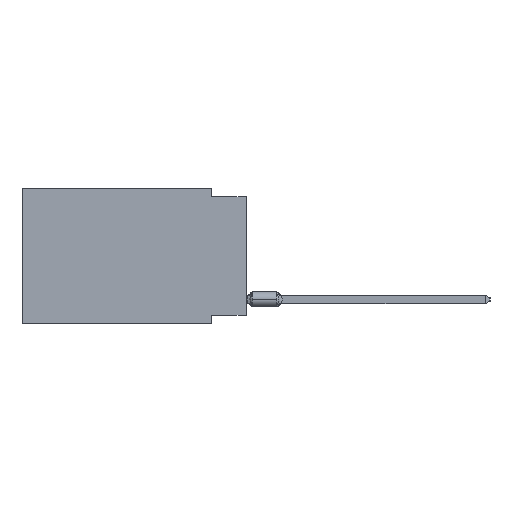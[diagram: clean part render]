
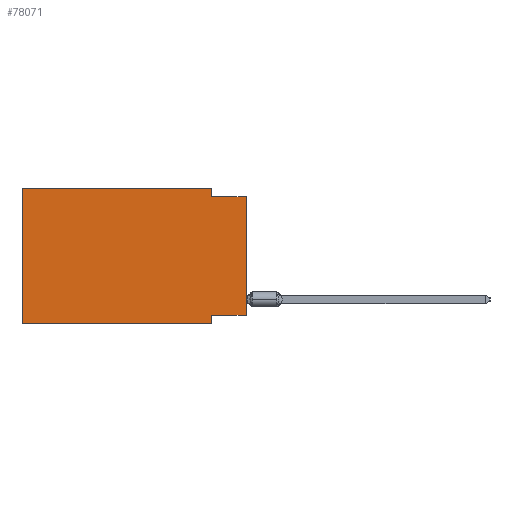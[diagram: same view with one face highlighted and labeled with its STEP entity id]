
A CAD part, left-side view. The second image highlights one B-rep face of the part: STEP entity #78071.
In plain terms, the highlighted planar face has unit normal (-1, 0, 0).
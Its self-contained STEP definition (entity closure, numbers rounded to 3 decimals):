
#1465 = EDGE_CURVE ( 'NONE', #5556, #40134, #46039, .T. ) ;
#3753 = CARTESIAN_POINT ( 'NONE',  ( 0., 2.54, -9.271 ) ) ;
#5556 = VERTEX_POINT ( 'NONE', #38442 ) ;
#6638 = EDGE_LOOP ( 'NONE', ( #44764, #62593, #68953, #17192, #56799, #29206, #59821, #19370 ) ) ;
#9472 = EDGE_CURVE ( 'NONE', #56695, #26319, #50409, .T. ) ;
#9802 = EDGE_CURVE ( 'NONE', #30794, #55463, #74869, .T. ) ;
#11977 = VECTOR ( 'NONE', #43719, 1000. ) ;
#12770 = CARTESIAN_POINT ( 'NONE',  ( 0., 16.383, -9.906 ) ) ;
#13799 = DIRECTION ( 'NONE',  ( 0., -1., 0. ) ) ;
#14411 = VERTEX_POINT ( 'NONE', #12770 ) ;
#15661 = EDGE_CURVE ( 'NONE', #40134, #53928, #49573, .T. ) ;
#17192 = ORIENTED_EDGE ( 'NONE', *, *, #9472, .F. ) ;
#19370 = ORIENTED_EDGE ( 'NONE', *, *, #1465, .F. ) ;
#23272 = CARTESIAN_POINT ( 'NONE',  ( 0., 0., 0. ) ) ;
#24877 = VECTOR ( 'NONE', #50468, 1000. ) ;
#25056 = DIRECTION ( 'NONE',  ( 0., 0., 1. ) ) ;
#26319 = VERTEX_POINT ( 'NONE', #87133 ) ;
#27004 = DIRECTION ( 'NONE',  ( 0., 0., -1. ) ) ;
#29206 = ORIENTED_EDGE ( 'NONE', *, *, #77268, .T. ) ;
#30794 = VERTEX_POINT ( 'NONE', #76246 ) ;
#32174 = LINE ( 'NONE', #64745, #60377 ) ;
#36394 = DIRECTION ( 'NONE',  ( 1., 0., 0. ) ) ;
#37855 = CARTESIAN_POINT ( 'NONE',  ( 0., 0., -0.635 ) ) ;
#38312 = CARTESIAN_POINT ( 'NONE',  ( 0., 16.383, 0. ) ) ;
#38442 = CARTESIAN_POINT ( 'NONE',  ( 0., 0., -9.271 ) ) ;
#40134 = VERTEX_POINT ( 'NONE', #3753 ) ;
#41725 = EDGE_CURVE ( 'NONE', #14411, #56695, #32174, .T. ) ;
#42622 = FACE_OUTER_BOUND ( 'NONE', #6638, .T. ) ;
#43304 = DIRECTION ( 'NONE',  ( 0., 0., -1. ) ) ;
#43719 = DIRECTION ( 'NONE',  ( 0., -1., 0. ) ) ;
#44764 = ORIENTED_EDGE ( 'NONE', *, *, #87607, .T. ) ;
#44879 = CARTESIAN_POINT ( 'NONE',  ( 0., 16.383, -9.906 ) ) ;
#46039 = LINE ( 'NONE', #87460, #70453 ) ;
#49573 = LINE ( 'NONE', #84270, #82880 ) ;
#50409 = LINE ( 'NONE', #84248, #11977 ) ;
#50468 = DIRECTION ( 'NONE',  ( 0., 0., 1. ) ) ;
#52006 = DIRECTION ( 'NONE',  ( 0., -1., 0. ) ) ;
#53928 = VERTEX_POINT ( 'NONE', #87074 ) ;
#54489 = DIRECTION ( 'NONE',  ( 0., 1., 0. ) ) ;
#55463 = VERTEX_POINT ( 'NONE', #37855 ) ;
#56695 = VERTEX_POINT ( 'NONE', #38312 ) ;
#56799 = ORIENTED_EDGE ( 'NONE', *, *, #41725, .F. ) ;
#59821 = ORIENTED_EDGE ( 'NONE', *, *, #15661, .F. ) ;
#60377 = VECTOR ( 'NONE', #25056, 1000. ) ;
#62593 = ORIENTED_EDGE ( 'NONE', *, *, #9802, .F. ) ;
#63188 = LINE ( 'NONE', #44879, #81735 ) ;
#64745 = CARTESIAN_POINT ( 'NONE',  ( 0., 16.383, 0. ) ) ;
#64782 = AXIS2_PLACEMENT_3D ( 'NONE', #70697, #36394, #83607 ) ;
#67568 = CARTESIAN_POINT ( 'NONE',  ( 0., 2.54, 0. ) ) ;
#68606 = CARTESIAN_POINT ( 'NONE',  ( 0., 0., -0.635 ) ) ;
#68953 = ORIENTED_EDGE ( 'NONE', *, *, #77549, .F. ) ;
#70453 = VECTOR ( 'NONE', #54489, 1000. ) ;
#70697 = CARTESIAN_POINT ( 'NONE',  ( 0., 16.383, 0. ) ) ;
#73262 = VECTOR ( 'NONE', #13799, 1000. ) ;
#74709 = VECTOR ( 'NONE', #27004, 1000. ) ;
#74869 = LINE ( 'NONE', #68606, #73262 ) ;
#76246 = CARTESIAN_POINT ( 'NONE',  ( 0., 2.54, -0.635 ) ) ;
#77268 = EDGE_CURVE ( 'NONE', #14411, #53928, #63188, .T. ) ;
#77368 = PLANE ( 'NONE',  #64782 ) ;
#77549 = EDGE_CURVE ( 'NONE', #26319, #30794, #80914, .T. ) ;
#78071 = ADVANCED_FACE ( 'NONE', ( #42622 ), #77368, .F. ) ;
#80914 = LINE ( 'NONE', #67568, #74709 ) ;
#81735 = VECTOR ( 'NONE', #52006, 1000. ) ;
#82880 = VECTOR ( 'NONE', #43304, 1000. ) ;
#83607 = DIRECTION ( 'NONE',  ( 0., 0., -1. ) ) ;
#84248 = CARTESIAN_POINT ( 'NONE',  ( 0., 16.383, 0. ) ) ;
#84270 = CARTESIAN_POINT ( 'NONE',  ( 0., 2.54, -9.906 ) ) ;
#84310 = LINE ( 'NONE', #23272, #24877 ) ;
#87074 = CARTESIAN_POINT ( 'NONE',  ( 0., 2.54, -9.906 ) ) ;
#87133 = CARTESIAN_POINT ( 'NONE',  ( 0., 2.54, 0. ) ) ;
#87460 = CARTESIAN_POINT ( 'NONE',  ( 0., 0., -9.271 ) ) ;
#87607 = EDGE_CURVE ( 'NONE', #5556, #55463, #84310, .T. ) ;
